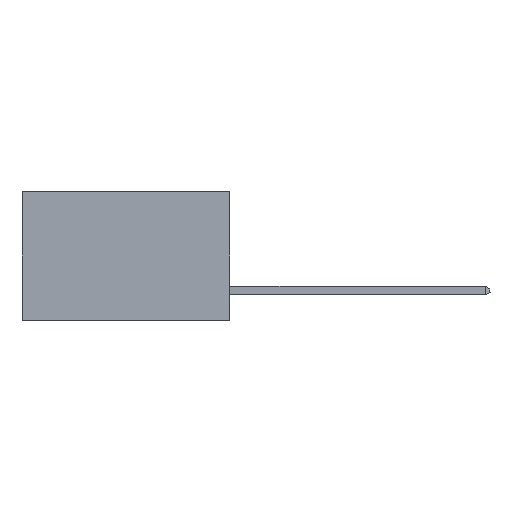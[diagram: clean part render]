
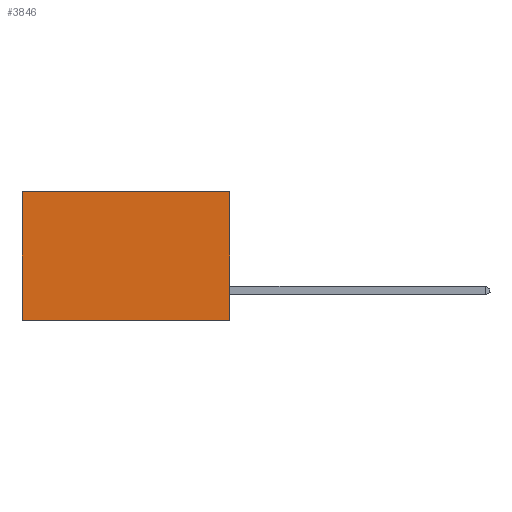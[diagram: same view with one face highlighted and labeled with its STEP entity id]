
A CAD part, left-side view. The second image highlights one B-rep face of the part: STEP entity #3846.
In plain terms, the highlighted planar face has unit normal (-1, 0, 0).
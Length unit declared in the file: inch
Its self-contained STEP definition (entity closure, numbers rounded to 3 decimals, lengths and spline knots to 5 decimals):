
#254 = EDGE_CURVE ( 'NONE', #3731, #6267, #10187, .T. ) ;
#420 = VECTOR ( 'NONE', #3134, 39.37008 ) ;
#494 = CARTESIAN_POINT ( 'NONE',  ( 0.298, 0., 0. ) ) ;
#913 = VERTEX_POINT ( 'NONE', #4659 ) ;
#961 = FACE_OUTER_BOUND ( 'NONE', #4883, .T. ) ;
#1399 = DIRECTION ( 'NONE',  ( 1., 0., 0. ) ) ;
#1565 = ORIENTED_EDGE ( 'NONE', *, *, #7361, .F. ) ;
#1592 = LINE ( 'NONE', #4578, #2159 ) ;
#2060 = EDGE_CURVE ( 'NONE', #3731, #913, #3213, .T. ) ;
#2159 = VECTOR ( 'NONE', #3789, 39.37008 ) ;
#2227 = PLANE ( 'NONE',  #7784 ) ;
#2399 = CARTESIAN_POINT ( 'NONE',  ( 0.298, 0., -0.37 ) ) ;
#3134 = DIRECTION ( 'NONE',  ( 0., 0., -1. ) ) ;
#3213 = LINE ( 'NONE', #4158, #10878 ) ;
#3226 = CARTESIAN_POINT ( 'NONE',  ( 0.298, 0.6, 0. ) ) ;
#3418 = VERTEX_POINT ( 'NONE', #6156 ) ;
#3731 = VERTEX_POINT ( 'NONE', #11067 ) ;
#3789 = DIRECTION ( 'NONE',  ( 0., 1., 0. ) ) ;
#3846 = ADVANCED_FACE ( 'NONE', ( #961 ), #2227, .F. ) ;
#3886 = CARTESIAN_POINT ( 'NONE',  ( 0.298, 0., 0. ) ) ;
#4158 = CARTESIAN_POINT ( 'NONE',  ( 0.298, 0., 0. ) ) ;
#4252 = LINE ( 'NONE', #3226, #8804 ) ;
#4578 = CARTESIAN_POINT ( 'NONE',  ( 0.298, 0., -0.37 ) ) ;
#4659 = CARTESIAN_POINT ( 'NONE',  ( 0.298, 0.6, 0. ) ) ;
#4883 = EDGE_LOOP ( 'NONE', ( #8583, #1565, #11629, #10427 ) ) ;
#6038 = DIRECTION ( 'NONE',  ( 0., 1., 0. ) ) ;
#6156 = CARTESIAN_POINT ( 'NONE',  ( 0.298, 0.6, -0.37 ) ) ;
#6267 = VERTEX_POINT ( 'NONE', #2399 ) ;
#6725 = EDGE_CURVE ( 'NONE', #913, #3418, #4252, .T. ) ;
#7361 = EDGE_CURVE ( 'NONE', #6267, #3418, #1592, .T. ) ;
#7784 = AXIS2_PLACEMENT_3D ( 'NONE', #494, #1399, #11376 ) ;
#8583 = ORIENTED_EDGE ( 'NONE', *, *, #6725, .T. ) ;
#8804 = VECTOR ( 'NONE', #9670, 39.37008 ) ;
#9670 = DIRECTION ( 'NONE',  ( 0., 0., -1. ) ) ;
#10187 = LINE ( 'NONE', #3886, #420 ) ;
#10427 = ORIENTED_EDGE ( 'NONE', *, *, #2060, .T. ) ;
#10878 = VECTOR ( 'NONE', #6038, 39.37008 ) ;
#11067 = CARTESIAN_POINT ( 'NONE',  ( 0.298, 0., 0. ) ) ;
#11376 = DIRECTION ( 'NONE',  ( 0., 0., -1. ) ) ;
#11629 = ORIENTED_EDGE ( 'NONE', *, *, #254, .F. ) ;
